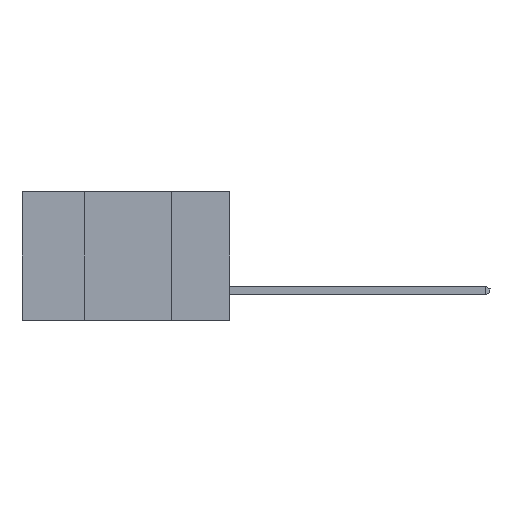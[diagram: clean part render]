
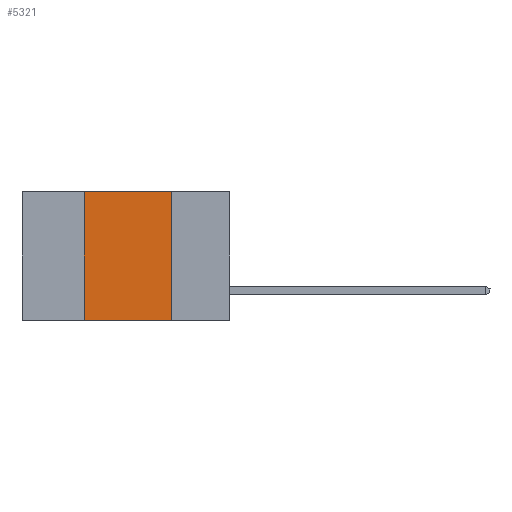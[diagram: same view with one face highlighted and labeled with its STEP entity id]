
A CAD part, left-side view. The second image highlights one B-rep face of the part: STEP entity #5321.
In plain terms, the highlighted planar face has unit normal (-1, 0, 0).
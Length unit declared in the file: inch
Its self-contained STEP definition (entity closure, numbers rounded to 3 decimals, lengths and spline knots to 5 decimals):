
#153 = CARTESIAN_POINT ( 'NONE',  ( 0., 0.42, -0.37 ) ) ;
#1009 = LINE ( 'NONE', #4551, #3985 ) ;
#1254 = VERTEX_POINT ( 'NONE', #11082 ) ;
#2469 = DIRECTION ( 'NONE',  ( 0., 0., -1. ) ) ;
#3575 = LINE ( 'NONE', #7177, #13829 ) ;
#3985 = VECTOR ( 'NONE', #2469, 39.37008 ) ;
#4111 = DIRECTION ( 'NONE',  ( 0., -1., 0. ) ) ;
#4551 = CARTESIAN_POINT ( 'NONE',  ( 0., 0.17, -0.37 ) ) ;
#4634 = EDGE_CURVE ( 'NONE', #12939, #11682, #11607, .T. ) ;
#5321 = ADVANCED_FACE ( 'NONE', ( #13602 ), #7800, .F. ) ;
#5425 = VECTOR ( 'NONE', #10448, 39.37008 ) ;
#5567 = CARTESIAN_POINT ( 'NONE',  ( 0., 0.6, 0. ) ) ;
#5613 = EDGE_LOOP ( 'NONE', ( #14060, #8853, #6001, #10689 ) ) ;
#5689 = AXIS2_PLACEMENT_3D ( 'NONE', #5567, #7729, #12506 ) ;
#5965 = VECTOR ( 'NONE', #4111, 39.37008 ) ;
#6001 = ORIENTED_EDGE ( 'NONE', *, *, #4634, .F. ) ;
#6402 = LINE ( 'NONE', #10182, #5965 ) ;
#6780 = CARTESIAN_POINT ( 'NONE',  ( 0., 0.42, 0. ) ) ;
#6862 = EDGE_CURVE ( 'NONE', #11682, #7756, #3575, .T. ) ;
#7177 = CARTESIAN_POINT ( 'NONE',  ( 0., 0.6, 0. ) ) ;
#7264 = EDGE_CURVE ( 'NONE', #7756, #1254, #1009, .T. ) ;
#7729 = DIRECTION ( 'NONE',  ( 1., 0., 0. ) ) ;
#7743 = CARTESIAN_POINT ( 'NONE',  ( 0., 0.17, 0. ) ) ;
#7756 = VERTEX_POINT ( 'NONE', #7743 ) ;
#7800 = PLANE ( 'NONE',  #5689 ) ;
#8853 = ORIENTED_EDGE ( 'NONE', *, *, #6862, .F. ) ;
#9807 = EDGE_CURVE ( 'NONE', #12939, #1254, #6402, .T. ) ;
#10182 = CARTESIAN_POINT ( 'NONE',  ( 0., 0.6, -0.37 ) ) ;
#10448 = DIRECTION ( 'NONE',  ( 0., 0., 1. ) ) ;
#10689 = ORIENTED_EDGE ( 'NONE', *, *, #9807, .T. ) ;
#11082 = CARTESIAN_POINT ( 'NONE',  ( 0., 0.17, -0.37 ) ) ;
#11607 = LINE ( 'NONE', #153, #5425 ) ;
#11682 = VERTEX_POINT ( 'NONE', #6780 ) ;
#11892 = DIRECTION ( 'NONE',  ( 0., -1., 0. ) ) ;
#12506 = DIRECTION ( 'NONE',  ( 0., 0., -1. ) ) ;
#12641 = CARTESIAN_POINT ( 'NONE',  ( 0., 0.42, -0.37 ) ) ;
#12939 = VERTEX_POINT ( 'NONE', #12641 ) ;
#13602 = FACE_OUTER_BOUND ( 'NONE', #5613, .T. ) ;
#13829 = VECTOR ( 'NONE', #11892, 39.37008 ) ;
#14060 = ORIENTED_EDGE ( 'NONE', *, *, #7264, .F. ) ;
